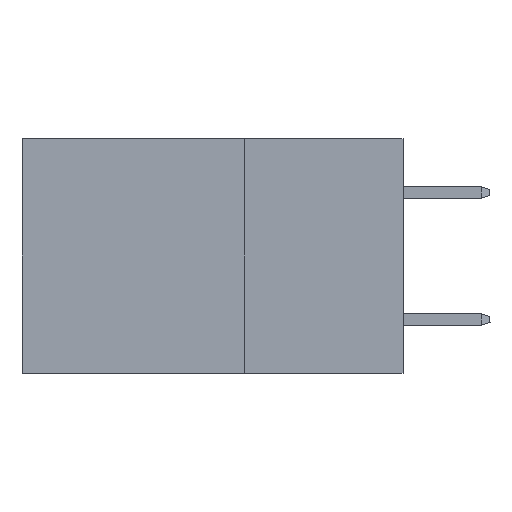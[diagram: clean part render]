
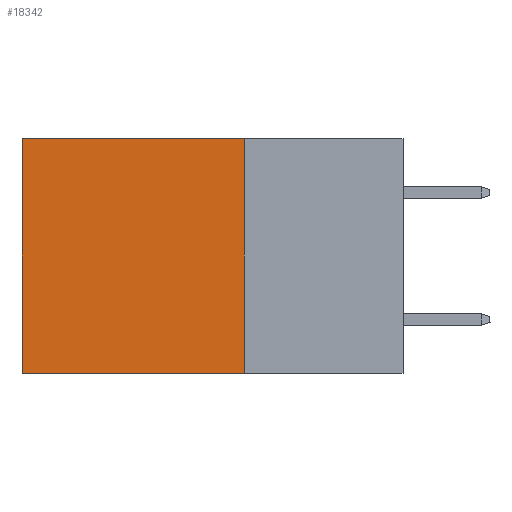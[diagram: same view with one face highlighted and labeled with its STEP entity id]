
A CAD part, left-side view. The second image highlights one B-rep face of the part: STEP entity #18342.
In plain terms, the highlighted planar face has unit normal (-1, 0, 0).
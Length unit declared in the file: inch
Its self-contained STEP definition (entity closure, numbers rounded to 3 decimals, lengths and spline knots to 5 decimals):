
#871 = ORIENTED_EDGE ( 'NONE', *, *, #23596, .F. ) ;
#910 = CARTESIAN_POINT ( 'NONE',  ( 0.2875, 0.6, 0. ) ) ;
#1640 = VECTOR ( 'NONE', #4281, 39.37008 ) ;
#1719 = PLANE ( 'NONE',  #5653 ) ;
#2862 = CARTESIAN_POINT ( 'NONE',  ( 0.2875, 0.25, -0.37 ) ) ;
#3393 = VERTEX_POINT ( 'NONE', #18178 ) ;
#4281 = DIRECTION ( 'NONE',  ( 0., 1., 0. ) ) ;
#4309 = CARTESIAN_POINT ( 'NONE',  ( 0.2875, 0.25, 0. ) ) ;
#5424 = CARTESIAN_POINT ( 'NONE',  ( 0.2875, 0.25, 0. ) ) ;
#5653 = AXIS2_PLACEMENT_3D ( 'NONE', #5424, #13475, #11555 ) ;
#5939 = ORIENTED_EDGE ( 'NONE', *, *, #19035, .T. ) ;
#6200 = VECTOR ( 'NONE', #19609, 39.37008 ) ;
#6542 = EDGE_CURVE ( 'NONE', #23310, #13002, #20394, .T. ) ;
#7272 = EDGE_CURVE ( 'NONE', #3393, #23093, #21577, .T. ) ;
#7501 = EDGE_LOOP ( 'NONE', ( #5939, #16740, #871, #8958 ) ) ;
#7589 = CARTESIAN_POINT ( 'NONE',  ( 0.2875, 0.25, 0. ) ) ;
#8958 = ORIENTED_EDGE ( 'NONE', *, *, #7272, .T. ) ;
#9513 = FACE_OUTER_BOUND ( 'NONE', #7501, .T. ) ;
#10560 = CARTESIAN_POINT ( 'NONE',  ( 0.2875, 0.25, -0.37 ) ) ;
#11555 = DIRECTION ( 'NONE',  ( 0., 0., -1. ) ) ;
#11855 = DIRECTION ( 'NONE',  ( 0., 1., 0. ) ) ;
#12102 = CARTESIAN_POINT ( 'NONE',  ( 0.2875, 0.6, 0. ) ) ;
#13002 = VERTEX_POINT ( 'NONE', #15281 ) ;
#13475 = DIRECTION ( 'NONE',  ( 1., 0., 0. ) ) ;
#14836 = LINE ( 'NONE', #910, #19530 ) ;
#15281 = CARTESIAN_POINT ( 'NONE',  ( 0.2875, 0.6, -0.37 ) ) ;
#16740 = ORIENTED_EDGE ( 'NONE', *, *, #6542, .F. ) ;
#17816 = LINE ( 'NONE', #7589, #6200 ) ;
#18178 = CARTESIAN_POINT ( 'NONE',  ( 0.2875, 0.25, 0. ) ) ;
#18342 = ADVANCED_FACE ( 'NONE', ( #9513 ), #1719, .F. ) ;
#19035 = EDGE_CURVE ( 'NONE', #23093, #13002, #14836, .T. ) ;
#19530 = VECTOR ( 'NONE', #22647, 39.37008 ) ;
#19609 = DIRECTION ( 'NONE',  ( 0., 0., -1. ) ) ;
#20394 = LINE ( 'NONE', #2862, #1640 ) ;
#21577 = LINE ( 'NONE', #4309, #22906 ) ;
#22647 = DIRECTION ( 'NONE',  ( 0., 0., -1. ) ) ;
#22906 = VECTOR ( 'NONE', #11855, 39.37008 ) ;
#23093 = VERTEX_POINT ( 'NONE', #12102 ) ;
#23310 = VERTEX_POINT ( 'NONE', #10560 ) ;
#23596 = EDGE_CURVE ( 'NONE', #3393, #23310, #17816, .T. ) ;
